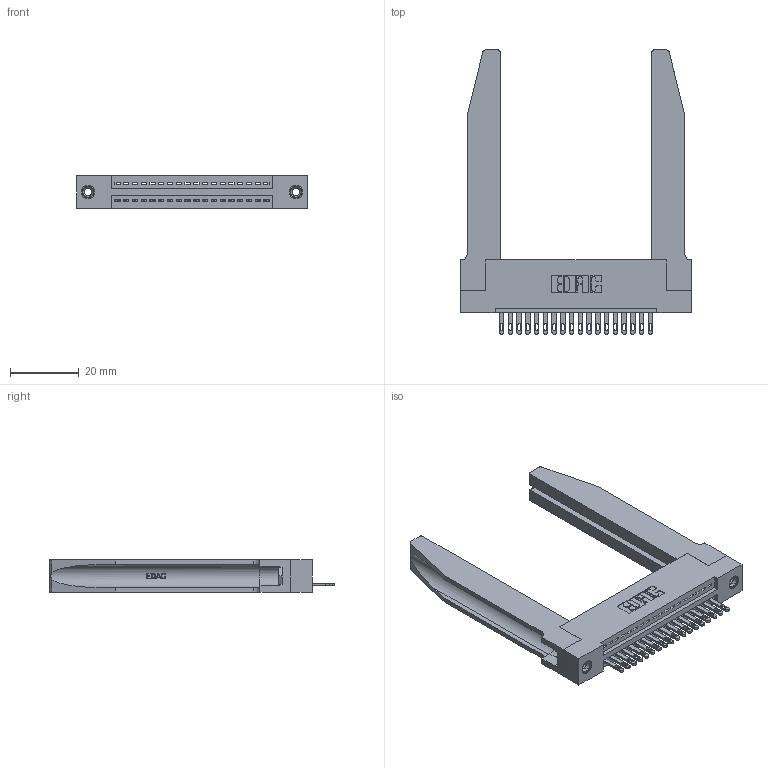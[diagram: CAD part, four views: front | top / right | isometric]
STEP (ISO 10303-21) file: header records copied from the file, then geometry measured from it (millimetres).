
FILE_DESCRIPTION (( 'STEP AP203' ), '1' );
FILE_NAME ('345-018-500-178.STEP', '2019-10-04T16:38:05', ( '' ), ( '' ), 'SwSTEP 2.0', 'SolidWorks 2016', '' );
FILE_SCHEMA (( 'CONFIG_CONTROL_DESIGN' ));
Length unit declared in the file: inch
Products named in the file (5): 345 Part_Flush Mounting Lugs - 0.156 Dia-TH; 345-292-001_345-293-100; 345-220-078_345-220-078; 345-018-500-178; 345-250-001_345-250-001-102
Assembly tree (23 placements, depth 2):
  345-018-500-178
    345 Part_Flush Mounting Lugs - 0.156 Dia-TH
    345-292-001_345-293-100  x18
    345-250-001_345-250-001-102  x2
    345-220-078_345-220-078  x2
Bounding box: 66.95 x 82.47 x 9.4 mm (x, y, z)
Volume: 13944.4 mm3; surface area: 14764.4 mm2
Topology: 23 solids, 23 shells, 1332 faces, 3973 edges, 2638 vertices
Faces by surface type: plane 834, cylinder 446, bspline 36, cone 12, torus 4
Entity records: 21448 total; most frequent: CARTESIAN_POINT 4613, ORIENTED_EDGE 3462, DIRECTION 3073, EDGE_CURVE 1731, VECTOR 1429, LINE 1429, VERTEX_POINT 1148, AXIS2_PLACEMENT_3D 822
